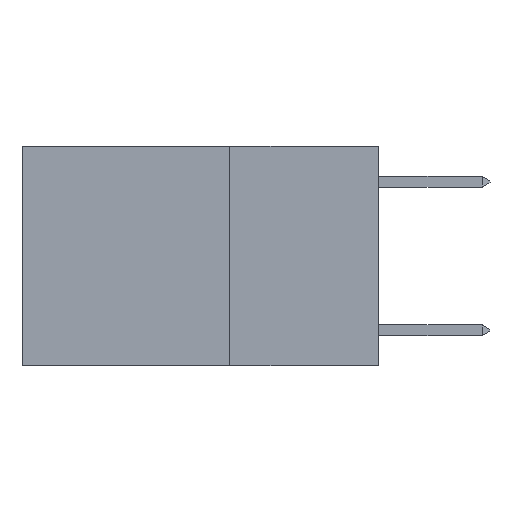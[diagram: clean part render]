
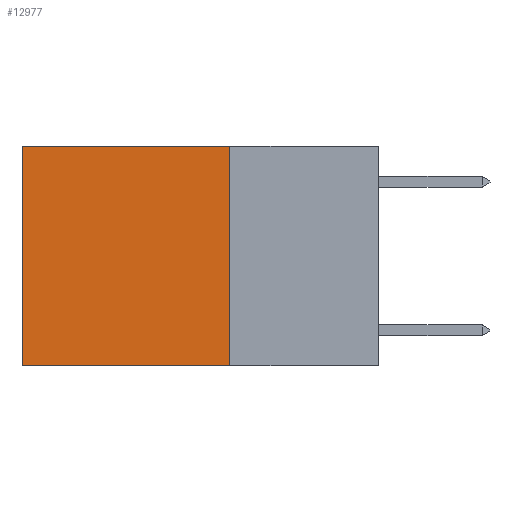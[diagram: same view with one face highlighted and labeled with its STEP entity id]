
A CAD part, left-side view. The second image highlights one B-rep face of the part: STEP entity #12977.
In plain terms, the highlighted planar face has unit normal (-1, 0, 0).
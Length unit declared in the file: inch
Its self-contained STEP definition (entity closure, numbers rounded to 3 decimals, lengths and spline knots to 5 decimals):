
#1835 = EDGE_LOOP ( 'NONE', ( #9999, #4147, #3547, #7238 ) ) ;
#2365 = VECTOR ( 'NONE', #10043, 39.37008 ) ;
#2838 = VERTEX_POINT ( 'NONE', #12028 ) ;
#3148 = CARTESIAN_POINT ( 'NONE',  ( 0.2625, 0.25, -0.37 ) ) ;
#3547 = ORIENTED_EDGE ( 'NONE', *, *, #9827, .F. ) ;
#3800 = VECTOR ( 'NONE', #8597, 39.37008 ) ;
#4147 = ORIENTED_EDGE ( 'NONE', *, *, #17242, .F. ) ;
#4192 = CARTESIAN_POINT ( 'NONE',  ( 0.2625, 0.25, -0.37 ) ) ;
#4756 = VERTEX_POINT ( 'NONE', #14823 ) ;
#5038 = LINE ( 'NONE', #10429, #8463 ) ;
#5300 = LINE ( 'NONE', #7179, #16422 ) ;
#6380 = DIRECTION ( 'NONE',  ( 1., 0., 0. ) ) ;
#7179 = CARTESIAN_POINT ( 'NONE',  ( 0.2625, 0.6, 0. ) ) ;
#7238 = ORIENTED_EDGE ( 'NONE', *, *, #17946, .T. ) ;
#7684 = CARTESIAN_POINT ( 'NONE',  ( 0.2625, 0.6, -0.37 ) ) ;
#8085 = FACE_OUTER_BOUND ( 'NONE', #1835, .T. ) ;
#8463 = VECTOR ( 'NONE', #13368, 39.37008 ) ;
#8597 = DIRECTION ( 'NONE',  ( 0., 1., 0. ) ) ;
#8622 = DIRECTION ( 'NONE',  ( 0., 0., -1. ) ) ;
#8907 = CARTESIAN_POINT ( 'NONE',  ( 0.2625, 0.25, 0. ) ) ;
#9140 = EDGE_CURVE ( 'NONE', #4756, #14982, #5300, .T. ) ;
#9827 = EDGE_CURVE ( 'NONE', #2838, #16271, #5038, .T. ) ;
#9999 = ORIENTED_EDGE ( 'NONE', *, *, #9140, .T. ) ;
#10043 = DIRECTION ( 'NONE',  ( 0., 1., 0. ) ) ;
#10429 = CARTESIAN_POINT ( 'NONE',  ( 0.2625, 0.25, 0. ) ) ;
#12028 = CARTESIAN_POINT ( 'NONE',  ( 0.2625, 0.25, 0. ) ) ;
#12237 = PLANE ( 'NONE',  #15406 ) ;
#12977 = ADVANCED_FACE ( 'NONE', ( #8085 ), #12237, .F. ) ;
#13368 = DIRECTION ( 'NONE',  ( 0., 0., -1. ) ) ;
#14823 = CARTESIAN_POINT ( 'NONE',  ( 0.2625, 0.6, 0. ) ) ;
#14982 = VERTEX_POINT ( 'NONE', #7684 ) ;
#15149 = CARTESIAN_POINT ( 'NONE',  ( 0.2625, 0.25, 0. ) ) ;
#15406 = AXIS2_PLACEMENT_3D ( 'NONE', #15149, #6380, #16538 ) ;
#15468 = LINE ( 'NONE', #4192, #3800 ) ;
#16271 = VERTEX_POINT ( 'NONE', #3148 ) ;
#16422 = VECTOR ( 'NONE', #8622, 39.37008 ) ;
#16538 = DIRECTION ( 'NONE',  ( 0., 0., -1. ) ) ;
#17242 = EDGE_CURVE ( 'NONE', #16271, #14982, #15468, .T. ) ;
#17420 = LINE ( 'NONE', #8907, #2365 ) ;
#17946 = EDGE_CURVE ( 'NONE', #2838, #4756, #17420, .T. ) ;
